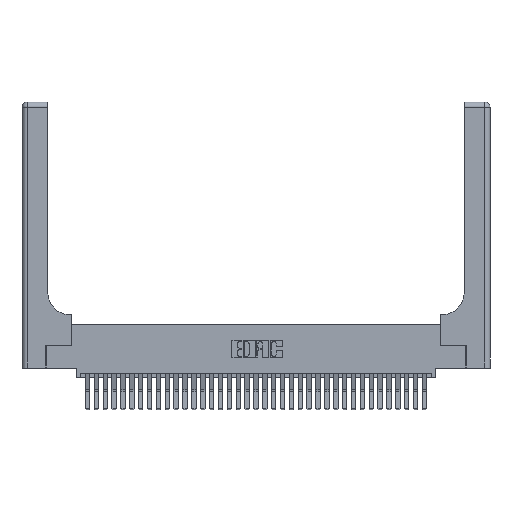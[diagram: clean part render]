
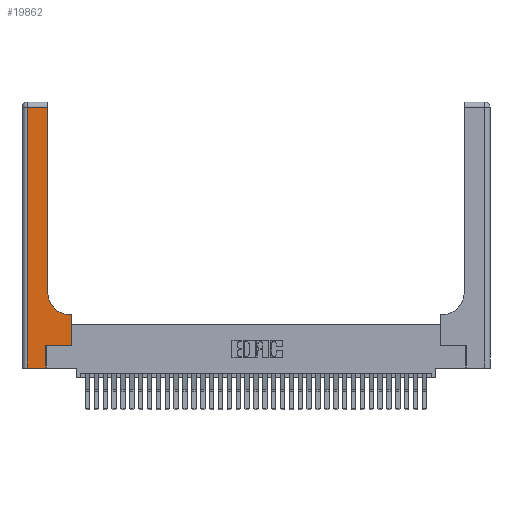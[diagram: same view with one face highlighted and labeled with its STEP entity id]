
A CAD part, top view. The second image highlights one B-rep face of the part: STEP entity #19862.
In plain terms, the highlighted planar face has unit normal (0, 0, 1).
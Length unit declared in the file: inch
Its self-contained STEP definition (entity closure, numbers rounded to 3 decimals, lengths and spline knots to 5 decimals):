
#234 = LINE ( 'NONE', #22505, #15452 ) ;
#360 = CARTESIAN_POINT ( 'NONE',  ( 0.5415, 0.85, 0.37 ) ) ;
#567 = DIRECTION ( 'NONE',  ( 1., 0., 0. ) ) ;
#590 = AXIS2_PLACEMENT_3D ( 'NONE', #360, #20258, #3262 ) ;
#1021 = VERTEX_POINT ( 'NONE', #8790 ) ;
#1067 = VERTEX_POINT ( 'NONE', #34172 ) ;
#2142 = DIRECTION ( 'NONE',  ( 0., 1., 0. ) ) ;
#2533 = DIRECTION ( 'NONE',  ( -1., 0., 0. ) ) ;
#3147 = CARTESIAN_POINT ( 'NONE',  ( 0., 2.94, 0.37 ) ) ;
#3262 = DIRECTION ( 'NONE',  ( 1., 0., 0. ) ) ;
#3565 = VECTOR ( 'NONE', #567, 39.37008 ) ;
#3981 = CIRCLE ( 'NONE', #590, 0.25 ) ;
#4801 = LINE ( 'NONE', #3147, #20740 ) ;
#6065 = LINE ( 'NONE', #10485, #18477 ) ;
#6137 = ORIENTED_EDGE ( 'NONE', *, *, #18517, .T. ) ;
#6197 = CARTESIAN_POINT ( 'NONE',  ( 0.2915, 0.85, 0.37 ) ) ;
#6362 = DIRECTION ( 'NONE',  ( -1., 0., 0. ) ) ;
#7481 = CARTESIAN_POINT ( 'NONE',  ( 0.5585, 0.6, 0.37 ) ) ;
#8525 = DIRECTION ( 'NONE',  ( 0., -1., 0. ) ) ;
#8790 = CARTESIAN_POINT ( 'NONE',  ( 0.06, 0., 0.37 ) ) ;
#8980 = VERTEX_POINT ( 'NONE', #16298 ) ;
#9752 = ORIENTED_EDGE ( 'NONE', *, *, #32979, .T. ) ;
#10330 = LINE ( 'NONE', #17656, #3565 ) ;
#10485 = CARTESIAN_POINT ( 'NONE',  ( 0.269, 0., 0.37 ) ) ;
#11119 = ORIENTED_EDGE ( 'NONE', *, *, #27043, .T. ) ;
#12257 = VERTEX_POINT ( 'NONE', #6197 ) ;
#12431 = ORIENTED_EDGE ( 'NONE', *, *, #34509, .T. ) ;
#12498 = CARTESIAN_POINT ( 'NONE',  ( 0.269, 0.25, 0.37 ) ) ;
#12886 = DIRECTION ( 'NONE',  ( 1., 0., 0. ) ) ;
#13312 = DIRECTION ( 'NONE',  ( 0., 1., 0. ) ) ;
#13451 = VERTEX_POINT ( 'NONE', #7481 ) ;
#13757 = ORIENTED_EDGE ( 'NONE', *, *, #25279, .T. ) ;
#14162 = DIRECTION ( 'NONE',  ( 0., 1., 0. ) ) ;
#14279 = FACE_OUTER_BOUND ( 'NONE', #29931, .T. ) ;
#14813 = VERTEX_POINT ( 'NONE', #16925 ) ;
#15452 = VECTOR ( 'NONE', #8525, 39.37008 ) ;
#15864 = LINE ( 'NONE', #35780, #30641 ) ;
#15948 = VERTEX_POINT ( 'NONE', #30850 ) ;
#16298 = CARTESIAN_POINT ( 'NONE',  ( 0.5415, 0.6, 0.37 ) ) ;
#16925 = CARTESIAN_POINT ( 'NONE',  ( 0.269, 0., 0.37 ) ) ;
#17526 = VECTOR ( 'NONE', #12886, 39.37008 ) ;
#17656 = CARTESIAN_POINT ( 'NONE',  ( 0.269, 0.25, 0.37 ) ) ;
#18477 = VECTOR ( 'NONE', #13312, 39.37008 ) ;
#18517 = EDGE_CURVE ( 'NONE', #12257, #1067, #27490, .T. ) ;
#18521 = CARTESIAN_POINT ( 'NONE',  ( 0., 0., 0.37 ) ) ;
#19254 = VECTOR ( 'NONE', #14162, 39.37008 ) ;
#19545 = DIRECTION ( 'NONE',  ( 0., 0., -1. ) ) ;
#19862 = ADVANCED_FACE ( 'NONE', ( #14279 ), #30578, .F. ) ;
#19981 = EDGE_CURVE ( 'NONE', #8980, #12257, #3981, .T. ) ;
#20258 = DIRECTION ( 'NONE',  ( 0., 0., -1. ) ) ;
#20740 = VECTOR ( 'NONE', #22908, 39.37008 ) ;
#22112 = EDGE_CURVE ( 'NONE', #30895, #13451, #15864, .T. ) ;
#22505 = CARTESIAN_POINT ( 'NONE',  ( 0.06, 3., 0.37 ) ) ;
#22908 = DIRECTION ( 'NONE',  ( -1., 0., 0. ) ) ;
#23225 = CARTESIAN_POINT ( 'NONE',  ( 0.2915, 0.6, 0.37 ) ) ;
#23751 = ORIENTED_EDGE ( 'NONE', *, *, #28591, .T. ) ;
#25279 = EDGE_CURVE ( 'NONE', #13451, #8980, #35732, .T. ) ;
#25743 = LINE ( 'NONE', #18521, #17526 ) ;
#27012 = CARTESIAN_POINT ( 'NONE',  ( 0.5585, 0.25, 0.37 ) ) ;
#27043 = EDGE_CURVE ( 'NONE', #31459, #30895, #10330, .T. ) ;
#27231 = ORIENTED_EDGE ( 'NONE', *, *, #33565, .T. ) ;
#27490 = LINE ( 'NONE', #28277, #19254 ) ;
#27792 = AXIS2_PLACEMENT_3D ( 'NONE', #36151, #19545, #2533 ) ;
#28277 = CARTESIAN_POINT ( 'NONE',  ( 0.2915, 3., 0.37 ) ) ;
#28573 = ORIENTED_EDGE ( 'NONE', *, *, #19981, .T. ) ;
#28591 = EDGE_CURVE ( 'NONE', #1067, #15948, #4801, .T. ) ;
#29239 = VECTOR ( 'NONE', #6362, 39.37008 ) ;
#29931 = EDGE_LOOP ( 'NONE', ( #6137, #23751, #9752, #12431, #27231, #11119, #33329, #13757, #28573 ) ) ;
#30578 = PLANE ( 'NONE',  #27792 ) ;
#30641 = VECTOR ( 'NONE', #2142, 39.37008 ) ;
#30850 = CARTESIAN_POINT ( 'NONE',  ( 0.06, 2.94, 0.37 ) ) ;
#30895 = VERTEX_POINT ( 'NONE', #27012 ) ;
#31459 = VERTEX_POINT ( 'NONE', #12498 ) ;
#32979 = EDGE_CURVE ( 'NONE', #15948, #1021, #234, .T. ) ;
#33329 = ORIENTED_EDGE ( 'NONE', *, *, #22112, .T. ) ;
#33565 = EDGE_CURVE ( 'NONE', #14813, #31459, #6065, .T. ) ;
#34172 = CARTESIAN_POINT ( 'NONE',  ( 0.2915, 2.94, 0.37 ) ) ;
#34509 = EDGE_CURVE ( 'NONE', #1021, #14813, #25743, .T. ) ;
#35732 = LINE ( 'NONE', #23225, #29239 ) ;
#35780 = CARTESIAN_POINT ( 'NONE',  ( 0.5585, 0.25, 0.37 ) ) ;
#36151 = CARTESIAN_POINT ( 'NONE',  ( 0., 3., 0.37 ) ) ;
